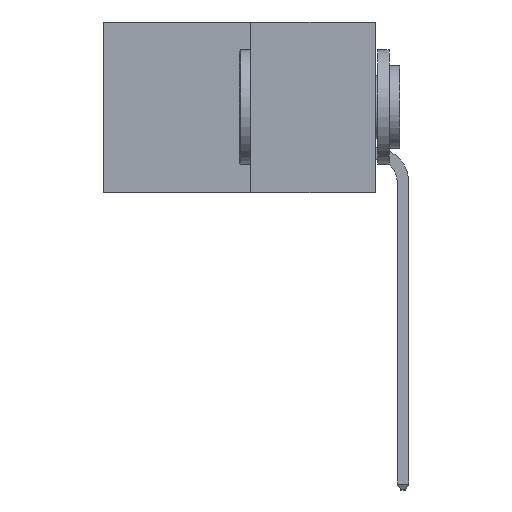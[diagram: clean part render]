
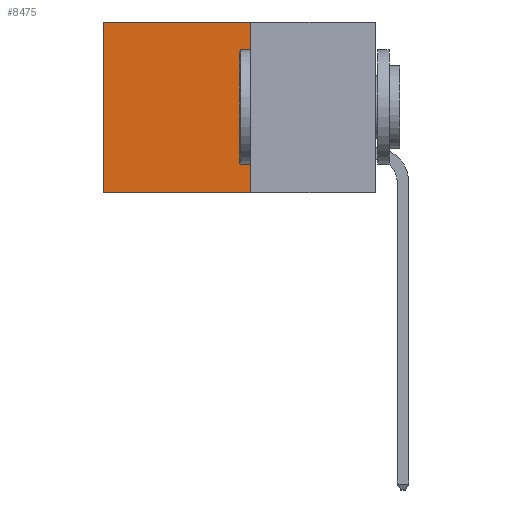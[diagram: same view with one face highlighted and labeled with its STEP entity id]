
A CAD part, left-side view. The second image highlights one B-rep face of the part: STEP entity #8475.
In plain terms, the highlighted planar face has unit normal (-1, 0, 0).
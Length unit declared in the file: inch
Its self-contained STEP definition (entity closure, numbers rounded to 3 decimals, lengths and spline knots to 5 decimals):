
#737 = DIRECTION ( 'NONE',  ( 1., 0., 0. ) ) ;
#2476 = VERTEX_POINT ( 'NONE', #17006 ) ;
#3042 = DIRECTION ( 'NONE',  ( 0., 1., 0. ) ) ;
#4555 = CARTESIAN_POINT ( 'NONE',  ( 0.277, 0.59, -0.37 ) ) ;
#5837 = VECTOR ( 'NONE', #3042, 39.37008 ) ;
#6089 = LINE ( 'NONE', #4555, #14827 ) ;
#6246 = ORIENTED_EDGE ( 'NONE', *, *, #6776, .F. ) ;
#6479 = DIRECTION ( 'NONE',  ( 0., 0., -1. ) ) ;
#6776 = EDGE_CURVE ( 'NONE', #22573, #2476, #23506, .T. ) ;
#7091 = DIRECTION ( 'NONE',  ( 0., 1., 0. ) ) ;
#7100 = CARTESIAN_POINT ( 'NONE',  ( 0.277, 0.27, -0.37 ) ) ;
#7650 = ORIENTED_EDGE ( 'NONE', *, *, #16836, .F. ) ;
#7803 = ORIENTED_EDGE ( 'NONE', *, *, #10255, .T. ) ;
#8475 = ADVANCED_FACE ( 'NONE', ( #17189 ), #19381, .F. ) ;
#8504 = ORIENTED_EDGE ( 'NONE', *, *, #14595, .T. ) ;
#8906 = VECTOR ( 'NONE', #7091, 39.37008 ) ;
#10255 = EDGE_CURVE ( 'NONE', #18555, #18071, #6089, .T. ) ;
#10791 = AXIS2_PLACEMENT_3D ( 'NONE', #12158, #737, #14050 ) ;
#12158 = CARTESIAN_POINT ( 'NONE',  ( 0.277, 0.27, -0.37 ) ) ;
#14050 = DIRECTION ( 'NONE',  ( 0., 0., -1. ) ) ;
#14310 = CARTESIAN_POINT ( 'NONE',  ( 0.277, 0.59, 0. ) ) ;
#14351 = CARTESIAN_POINT ( 'NONE',  ( 0.277, 0.27, -0.37 ) ) ;
#14595 = EDGE_CURVE ( 'NONE', #22573, #18555, #23272, .T. ) ;
#14827 = VECTOR ( 'NONE', #6479, 39.37008 ) ;
#15756 = LINE ( 'NONE', #14351, #5837 ) ;
#16331 = DIRECTION ( 'NONE',  ( 0., 0., -1. ) ) ;
#16836 = EDGE_CURVE ( 'NONE', #2476, #18071, #15756, .T. ) ;
#17006 = CARTESIAN_POINT ( 'NONE',  ( 0.277, 0.27, -0.37 ) ) ;
#17135 = CARTESIAN_POINT ( 'NONE',  ( 0.277, 0.27, 0. ) ) ;
#17189 = FACE_OUTER_BOUND ( 'NONE', #21925, .T. ) ;
#18071 = VERTEX_POINT ( 'NONE', #19777 ) ;
#18555 = VERTEX_POINT ( 'NONE', #14310 ) ;
#18887 = VECTOR ( 'NONE', #16331, 39.37008 ) ;
#19381 = PLANE ( 'NONE',  #10791 ) ;
#19777 = CARTESIAN_POINT ( 'NONE',  ( 0.277, 0.59, -0.37 ) ) ;
#19897 = CARTESIAN_POINT ( 'NONE',  ( 0.277, 0.27, 0. ) ) ;
#21925 = EDGE_LOOP ( 'NONE', ( #7803, #7650, #6246, #8504 ) ) ;
#22573 = VERTEX_POINT ( 'NONE', #17135 ) ;
#23272 = LINE ( 'NONE', #19897, #8906 ) ;
#23506 = LINE ( 'NONE', #7100, #18887 ) ;
